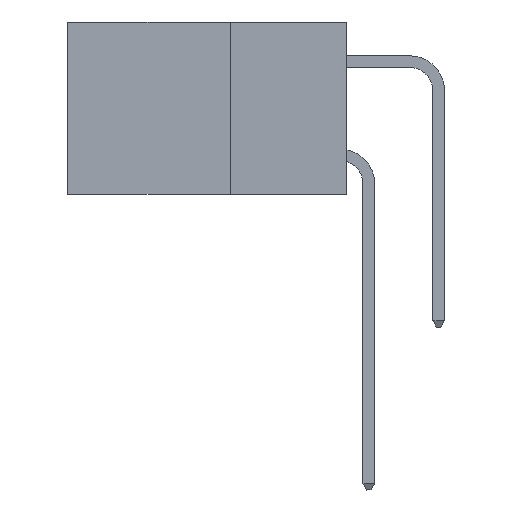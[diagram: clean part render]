
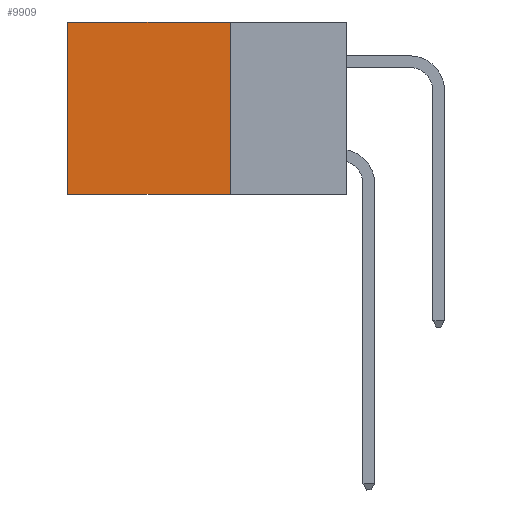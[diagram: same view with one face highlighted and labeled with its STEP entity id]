
A CAD part, left-side view. The second image highlights one B-rep face of the part: STEP entity #9909.
In plain terms, the highlighted planar face has unit normal (-1, 0, 0).
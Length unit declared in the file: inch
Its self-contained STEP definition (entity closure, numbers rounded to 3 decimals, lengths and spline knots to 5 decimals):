
#785 = DIRECTION ( 'NONE',  ( 0., 1., 0. ) ) ;
#794 = CARTESIAN_POINT ( 'NONE',  ( 0.2875, 0.6, 0. ) ) ;
#1541 = ORIENTED_EDGE ( 'NONE', *, *, #11590, .F. ) ;
#1789 = CARTESIAN_POINT ( 'NONE',  ( 0.2875, 0.6, -0.37 ) ) ;
#4265 = DIRECTION ( 'NONE',  ( 0., 0., -1. ) ) ;
#4318 = VECTOR ( 'NONE', #785, 39.37008 ) ;
#6511 = VECTOR ( 'NONE', #4265, 39.37008 ) ;
#6737 = DIRECTION ( 'NONE',  ( 0., 0., -1. ) ) ;
#9332 = DIRECTION ( 'NONE',  ( 0., 0., -1. ) ) ;
#9909 = ADVANCED_FACE ( 'NONE', ( #26672 ), #20047, .F. ) ;
#11590 = EDGE_CURVE ( 'NONE', #22599, #24973, #33332, .T. ) ;
#12134 = CARTESIAN_POINT ( 'NONE',  ( 0.2875, 0.25, -0.37 ) ) ;
#12221 = CARTESIAN_POINT ( 'NONE',  ( 0.2875, 0.25, 0. ) ) ;
#15380 = VERTEX_POINT ( 'NONE', #1789 ) ;
#15604 = AXIS2_PLACEMENT_3D ( 'NONE', #25275, #19376, #9332 ) ;
#16688 = VERTEX_POINT ( 'NONE', #794 ) ;
#17081 = CARTESIAN_POINT ( 'NONE',  ( 0.2875, 0.25, 0. ) ) ;
#17781 = ORIENTED_EDGE ( 'NONE', *, *, #28927, .T. ) ;
#18661 = EDGE_LOOP ( 'NONE', ( #17781, #24475, #1541, #34507 ) ) ;
#18775 = LINE ( 'NONE', #31234, #33446 ) ;
#19376 = DIRECTION ( 'NONE',  ( 1., 0., 0. ) ) ;
#20047 = PLANE ( 'NONE',  #15604 ) ;
#21945 = LINE ( 'NONE', #28428, #23413 ) ;
#22260 = EDGE_CURVE ( 'NONE', #24973, #15380, #18775, .T. ) ;
#22599 = VERTEX_POINT ( 'NONE', #12221 ) ;
#23413 = VECTOR ( 'NONE', #6737, 39.37008 ) ;
#24475 = ORIENTED_EDGE ( 'NONE', *, *, #22260, .F. ) ;
#24973 = VERTEX_POINT ( 'NONE', #12134 ) ;
#25275 = CARTESIAN_POINT ( 'NONE',  ( 0.2875, 0.25, 0. ) ) ;
#26672 = FACE_OUTER_BOUND ( 'NONE', #18661, .T. ) ;
#28428 = CARTESIAN_POINT ( 'NONE',  ( 0.2875, 0.6, 0. ) ) ;
#28927 = EDGE_CURVE ( 'NONE', #16688, #15380, #21945, .T. ) ;
#29119 = EDGE_CURVE ( 'NONE', #22599, #16688, #38465, .T. ) ;
#31234 = CARTESIAN_POINT ( 'NONE',  ( 0.2875, 0.25, -0.37 ) ) ;
#33332 = LINE ( 'NONE', #17081, #6511 ) ;
#33446 = VECTOR ( 'NONE', #33669, 39.37008 ) ;
#33669 = DIRECTION ( 'NONE',  ( 0., 1., 0. ) ) ;
#34507 = ORIENTED_EDGE ( 'NONE', *, *, #29119, .T. ) ;
#38465 = LINE ( 'NONE', #38467, #4318 ) ;
#38467 = CARTESIAN_POINT ( 'NONE',  ( 0.2875, 0.25, 0. ) ) ;
